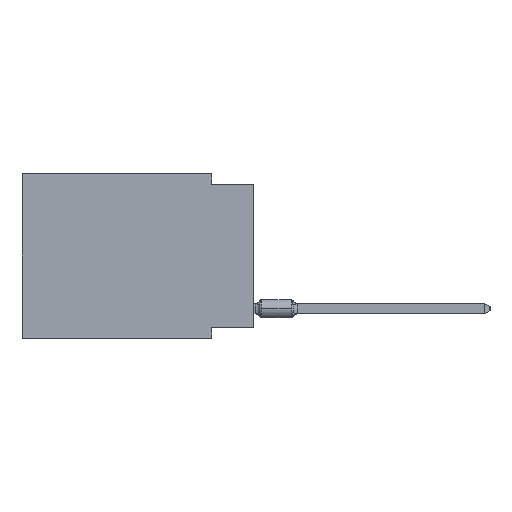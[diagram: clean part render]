
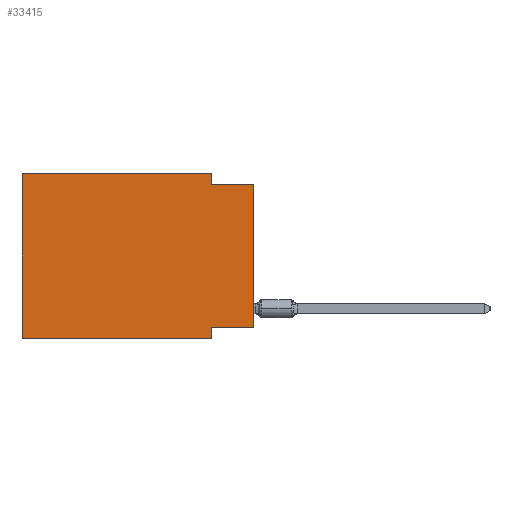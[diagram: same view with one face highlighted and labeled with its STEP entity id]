
A CAD part, left-side view. The second image highlights one B-rep face of the part: STEP entity #33415.
In plain terms, the highlighted planar face has unit normal (-1, 0, 0).
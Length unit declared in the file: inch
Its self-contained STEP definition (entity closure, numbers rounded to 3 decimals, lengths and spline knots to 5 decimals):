
#202 = EDGE_CURVE ( 'NONE', #61627, #7681, #1308, .T. ) ;
#1283 = CARTESIAN_POINT ( 'NONE',  ( 0., 0.55, -0.39 ) ) ;
#1308 = LINE ( 'NONE', #32442, #26449 ) ;
#2291 = VERTEX_POINT ( 'NONE', #16638 ) ;
#2621 = CARTESIAN_POINT ( 'NONE',  ( 0., 0.55, 0. ) ) ;
#3569 = VECTOR ( 'NONE', #52911, 39.37008 ) ;
#5442 = VERTEX_POINT ( 'NONE', #33347 ) ;
#5957 = CARTESIAN_POINT ( 'NONE',  ( 0., 0.1, -0.39 ) ) ;
#6816 = EDGE_CURVE ( 'NONE', #61627, #40462, #20932, .T. ) ;
#7000 = CARTESIAN_POINT ( 'NONE',  ( 0., 0.1, 0. ) ) ;
#7681 = VERTEX_POINT ( 'NONE', #36500 ) ;
#9201 = LINE ( 'NONE', #9857, #24882 ) ;
#9857 = CARTESIAN_POINT ( 'NONE',  ( 0., 0.55, 0. ) ) ;
#10870 = CARTESIAN_POINT ( 'NONE',  ( 0., 0., -0.365 ) ) ;
#11634 = EDGE_CURVE ( 'NONE', #36904, #53054, #51697, .T. ) ;
#12478 = CARTESIAN_POINT ( 'NONE',  ( 0., 0., -0.365 ) ) ;
#13533 = DIRECTION ( 'NONE',  ( 0., 0., -1. ) ) ;
#16445 = FACE_OUTER_BOUND ( 'NONE', #35416, .T. ) ;
#16638 = CARTESIAN_POINT ( 'NONE',  ( 0., 0.1, 0. ) ) ;
#16758 = LINE ( 'NONE', #57622, #48650 ) ;
#17895 = ORIENTED_EDGE ( 'NONE', *, *, #22402, .F. ) ;
#18201 = EDGE_CURVE ( 'NONE', #40122, #7681, #58487, .T. ) ;
#19153 = ORIENTED_EDGE ( 'NONE', *, *, #47061, .F. ) ;
#20932 = LINE ( 'NONE', #10870, #58352 ) ;
#21741 = DIRECTION ( 'NONE',  ( 0., 0., 1. ) ) ;
#22402 = EDGE_CURVE ( 'NONE', #2291, #40122, #58895, .T. ) ;
#24882 = VECTOR ( 'NONE', #66110, 39.37008 ) ;
#26220 = CARTESIAN_POINT ( 'NONE',  ( 0., 0.55, -0.39 ) ) ;
#26449 = VECTOR ( 'NONE', #21741, 39.37008 ) ;
#28112 = ORIENTED_EDGE ( 'NONE', *, *, #18201, .F. ) ;
#30317 = ORIENTED_EDGE ( 'NONE', *, *, #202, .T. ) ;
#32442 = CARTESIAN_POINT ( 'NONE',  ( 0., 0., 0. ) ) ;
#33347 = CARTESIAN_POINT ( 'NONE',  ( 0., 0.55, 0. ) ) ;
#33415 = ADVANCED_FACE ( 'NONE', ( #16445 ), #43789, .F. ) ;
#33620 = CARTESIAN_POINT ( 'NONE',  ( 0., 0.1, -0.39 ) ) ;
#35416 = EDGE_LOOP ( 'NONE', ( #30317, #28112, #17895, #42950, #66216, #51744, #19153, #61074 ) ) ;
#36500 = CARTESIAN_POINT ( 'NONE',  ( 0., 0., -0.025 ) ) ;
#36904 = VERTEX_POINT ( 'NONE', #1283 ) ;
#37101 = CARTESIAN_POINT ( 'NONE',  ( 0., 0.1, -0.365 ) ) ;
#38372 = DIRECTION ( 'NONE',  ( 0., -1., 0. ) ) ;
#38765 = DIRECTION ( 'NONE',  ( 0., 0., -1. ) ) ;
#39303 = LINE ( 'NONE', #33620, #59982 ) ;
#39689 = VECTOR ( 'NONE', #38372, 39.37008 ) ;
#40122 = VERTEX_POINT ( 'NONE', #52596 ) ;
#40462 = VERTEX_POINT ( 'NONE', #37101 ) ;
#40690 = DIRECTION ( 'NONE',  ( 0., 1., 0. ) ) ;
#42950 = ORIENTED_EDGE ( 'NONE', *, *, #60051, .F. ) ;
#43789 = PLANE ( 'NONE',  #55524 ) ;
#44988 = CARTESIAN_POINT ( 'NONE',  ( 0., 0., -0.025 ) ) ;
#46660 = DIRECTION ( 'NONE',  ( 0., -1., 0. ) ) ;
#47061 = EDGE_CURVE ( 'NONE', #40462, #53054, #39303, .T. ) ;
#48650 = VECTOR ( 'NONE', #56981, 39.37008 ) ;
#51697 = LINE ( 'NONE', #26220, #64213 ) ;
#51744 = ORIENTED_EDGE ( 'NONE', *, *, #11634, .T. ) ;
#52596 = CARTESIAN_POINT ( 'NONE',  ( 0., 0.1, -0.025 ) ) ;
#52911 = DIRECTION ( 'NONE',  ( 0., 0., -1. ) ) ;
#53054 = VERTEX_POINT ( 'NONE', #5957 ) ;
#55524 = AXIS2_PLACEMENT_3D ( 'NONE', #2621, #64200, #38765 ) ;
#56981 = DIRECTION ( 'NONE',  ( 0., -1., 0. ) ) ;
#57622 = CARTESIAN_POINT ( 'NONE',  ( 0., 0.55, 0. ) ) ;
#57786 = EDGE_CURVE ( 'NONE', #36904, #5442, #9201, .T. ) ;
#58352 = VECTOR ( 'NONE', #40690, 39.37008 ) ;
#58487 = LINE ( 'NONE', #44988, #39689 ) ;
#58895 = LINE ( 'NONE', #7000, #3569 ) ;
#59982 = VECTOR ( 'NONE', #13533, 39.37008 ) ;
#60051 = EDGE_CURVE ( 'NONE', #5442, #2291, #16758, .T. ) ;
#61074 = ORIENTED_EDGE ( 'NONE', *, *, #6816, .F. ) ;
#61627 = VERTEX_POINT ( 'NONE', #12478 ) ;
#64200 = DIRECTION ( 'NONE',  ( 1., 0., 0. ) ) ;
#64213 = VECTOR ( 'NONE', #46660, 39.37008 ) ;
#66110 = DIRECTION ( 'NONE',  ( 0., 0., 1. ) ) ;
#66216 = ORIENTED_EDGE ( 'NONE', *, *, #57786, .F. ) ;
